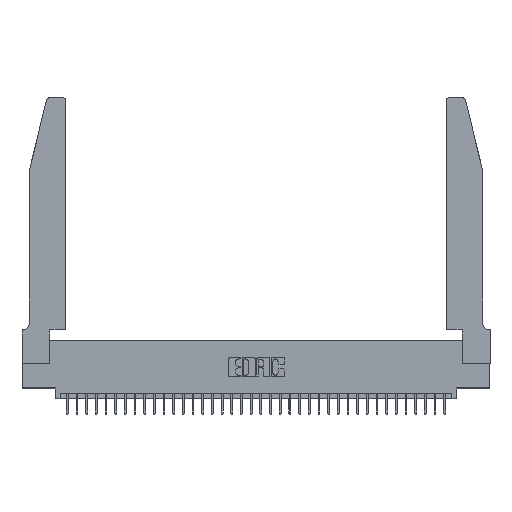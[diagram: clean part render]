
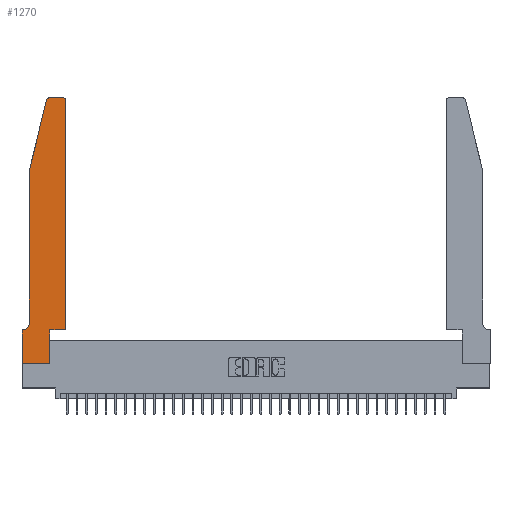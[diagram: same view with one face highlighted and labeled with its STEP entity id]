
A CAD part, top view. The second image highlights one B-rep face of the part: STEP entity #1270.
In plain terms, the highlighted planar face has unit normal (0, 0, 1).
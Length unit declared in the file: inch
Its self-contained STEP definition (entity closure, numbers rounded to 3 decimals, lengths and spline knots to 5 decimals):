
#65 = EDGE_CURVE ( 'NONE', #24321, #22685, #24032, .T. ) ;
#517 = EDGE_CURVE ( 'NONE', #23599, #31405, #6212, .T. ) ;
#1083 = EDGE_CURVE ( 'NONE', #31405, #13949, #21759, .T. ) ;
#1270 = ADVANCED_FACE ( 'NONE', ( #4887 ), #7779, .T. ) ;
#1396 = DIRECTION ( 'NONE',  ( 0., 0., 1. ) ) ;
#2242 = DIRECTION ( 'NONE',  ( 0., -1., 0. ) ) ;
#2376 = VERTEX_POINT ( 'NONE', #35220 ) ;
#2506 = LINE ( 'NONE', #8775, #5583 ) ;
#4100 = ORIENTED_EDGE ( 'NONE', *, *, #517, .T. ) ;
#4130 = EDGE_CURVE ( 'NONE', #23482, #27998, #27490, .T. ) ;
#4410 = EDGE_CURVE ( 'NONE', #2376, #6385, #9303, .T. ) ;
#4876 = LINE ( 'NONE', #26393, #8856 ) ;
#4887 = FACE_OUTER_BOUND ( 'NONE', #32056, .T. ) ;
#5583 = VECTOR ( 'NONE', #20606, 39.37008 ) ;
#5746 = ORIENTED_EDGE ( 'NONE', *, *, #16310, .T. ) ;
#6212 = CIRCLE ( 'NONE', #23201, 0.03 ) ;
#6385 = VERTEX_POINT ( 'NONE', #10218 ) ;
#6633 = VECTOR ( 'NONE', #18311, 39.37008 ) ;
#6755 = ORIENTED_EDGE ( 'NONE', *, *, #4410, .T. ) ;
#6871 = CARTESIAN_POINT ( 'NONE',  ( 0.4205, 2.75, 0.37 ) ) ;
#7328 = LINE ( 'NONE', #31732, #21506 ) ;
#7779 = PLANE ( 'NONE',  #19932 ) ;
#7938 = VECTOR ( 'NONE', #24147, 39.37008 ) ;
#8775 = CARTESIAN_POINT ( 'NONE',  ( 0., 0., 0.37 ) ) ;
#8856 = VECTOR ( 'NONE', #24224, 39.37008 ) ;
#9303 = LINE ( 'NONE', #9521, #28753 ) ;
#9521 = CARTESIAN_POINT ( 'NONE',  ( 0.2865, 0.35, 0.37 ) ) ;
#9936 = CARTESIAN_POINT ( 'NONE',  ( 0.0755, 2., 0.37 ) ) ;
#10218 = CARTESIAN_POINT ( 'NONE',  ( 0.2865, 0.35, 0.37 ) ) ;
#10631 = CARTESIAN_POINT ( 'NONE',  ( 0., 0.35, 0.37 ) ) ;
#10821 = CARTESIAN_POINT ( 'NONE',  ( 0.0055, 0.42, 0.37 ) ) ;
#11237 = CARTESIAN_POINT ( 'NONE',  ( 0.0755, 2., 0.37 ) ) ;
#11319 = EDGE_CURVE ( 'NONE', #13949, #31906, #30739, .T. ) ;
#13082 = ORIENTED_EDGE ( 'NONE', *, *, #11319, .T. ) ;
#13360 = EDGE_CURVE ( 'NONE', #6385, #20041, #4876, .T. ) ;
#13949 = VERTEX_POINT ( 'NONE', #18133 ) ;
#14176 = CARTESIAN_POINT ( 'NONE',  ( 0.284, 2.75, 0.37 ) ) ;
#14812 = DIRECTION ( 'NONE',  ( -1., 0., 0. ) ) ;
#15260 = CARTESIAN_POINT ( 'NONE',  ( 0.4205, 2.72, 0.37 ) ) ;
#15586 = CARTESIAN_POINT ( 'NONE',  ( 0.0755, 0.35, 0.37 ) ) ;
#16310 = EDGE_CURVE ( 'NONE', #19633, #24321, #23368, .T. ) ;
#16917 = ORIENTED_EDGE ( 'NONE', *, *, #17062, .T. ) ;
#17062 = EDGE_CURVE ( 'NONE', #31906, #19633, #22103, .T. ) ;
#17596 = CARTESIAN_POINT ( 'NONE',  ( 0.0055, 0.35, 0.37 ) ) ;
#18133 = CARTESIAN_POINT ( 'NONE',  ( 0.0755, 2., 0.37 ) ) ;
#18311 = DIRECTION ( 'NONE',  ( -0.239, -0.971, 0. ) ) ;
#18563 = ORIENTED_EDGE ( 'NONE', *, *, #35576, .T. ) ;
#19015 = DIRECTION ( 'NONE',  ( 1., 0., 0. ) ) ;
#19085 = CARTESIAN_POINT ( 'NONE',  ( 0.4505, 0.35, 0.37 ) ) ;
#19585 = ORIENTED_EDGE ( 'NONE', *, *, #28231, .T. ) ;
#19633 = VERTEX_POINT ( 'NONE', #17596 ) ;
#19932 = AXIS2_PLACEMENT_3D ( 'NONE', #10631, #30389, #24846 ) ;
#19980 = AXIS2_PLACEMENT_3D ( 'NONE', #15260, #1396, #20960 ) ;
#20041 = VERTEX_POINT ( 'NONE', #28250 ) ;
#20606 = DIRECTION ( 'NONE',  ( 1., 0., 0. ) ) ;
#20960 = DIRECTION ( 'NONE',  ( 1., 0., 0. ) ) ;
#21506 = VECTOR ( 'NONE', #14812, 39.37008 ) ;
#21719 = DIRECTION ( 'NONE',  ( 0., 0., 1. ) ) ;
#21759 = LINE ( 'NONE', #11237, #6633 ) ;
#21863 = VECTOR ( 'NONE', #26965, 39.37008 ) ;
#22103 = CIRCLE ( 'NONE', #25994, 0.07 ) ;
#22685 = VERTEX_POINT ( 'NONE', #27129 ) ;
#23062 = ORIENTED_EDGE ( 'NONE', *, *, #65, .T. ) ;
#23201 = AXIS2_PLACEMENT_3D ( 'NONE', #35935, #21719, #19015 ) ;
#23368 = LINE ( 'NONE', #15586, #7938 ) ;
#23482 = VERTEX_POINT ( 'NONE', #25047 ) ;
#23599 = VERTEX_POINT ( 'NONE', #14176 ) ;
#23753 = VECTOR ( 'NONE', #33496, 39.37008 ) ;
#23777 = CARTESIAN_POINT ( 'NONE',  ( 0.25487, 2.72718, 0.37 ) ) ;
#24032 = LINE ( 'NONE', #35871, #31125 ) ;
#24147 = DIRECTION ( 'NONE',  ( -1., 0., 0. ) ) ;
#24224 = DIRECTION ( 'NONE',  ( 1., 0., 0. ) ) ;
#24321 = VERTEX_POINT ( 'NONE', #36551 ) ;
#24846 = DIRECTION ( 'NONE',  ( 1., 0., 0. ) ) ;
#25047 = CARTESIAN_POINT ( 'NONE',  ( 0.4505, 2.72, 0.37 ) ) ;
#25326 = ORIENTED_EDGE ( 'NONE', *, *, #33164, .T. ) ;
#25994 = AXIS2_PLACEMENT_3D ( 'NONE', #10821, #30830, #33272 ) ;
#26393 = CARTESIAN_POINT ( 'NONE',  ( 0.4505, 0.35, 0.37 ) ) ;
#26965 = DIRECTION ( 'NONE',  ( 0., -1., 0. ) ) ;
#27129 = CARTESIAN_POINT ( 'NONE',  ( 0., 0., 0.37 ) ) ;
#27490 = CIRCLE ( 'NONE', #19980, 0.03 ) ;
#27998 = VERTEX_POINT ( 'NONE', #6871 ) ;
#28231 = EDGE_CURVE ( 'NONE', #20041, #23482, #34776, .T. ) ;
#28250 = CARTESIAN_POINT ( 'NONE',  ( 0.4505, 0.35, 0.37 ) ) ;
#28753 = VECTOR ( 'NONE', #35430, 39.37008 ) ;
#28917 = CARTESIAN_POINT ( 'NONE',  ( 0.0755, 0.42, 0.37 ) ) ;
#30389 = DIRECTION ( 'NONE',  ( 0., 0., 1. ) ) ;
#30739 = LINE ( 'NONE', #9936, #21863 ) ;
#30830 = DIRECTION ( 'NONE',  ( 0., 0., -1. ) ) ;
#31125 = VECTOR ( 'NONE', #2242, 39.37008 ) ;
#31405 = VERTEX_POINT ( 'NONE', #23777 ) ;
#31732 = CARTESIAN_POINT ( 'NONE',  ( 0.2605, 2.75, 0.37 ) ) ;
#31906 = VERTEX_POINT ( 'NONE', #28917 ) ;
#32056 = EDGE_LOOP ( 'NONE', ( #25326, #4100, #34082, #13082, #16917, #5746, #23062, #18563, #6755, #35699, #19585, #32792 ) ) ;
#32792 = ORIENTED_EDGE ( 'NONE', *, *, #4130, .T. ) ;
#33164 = EDGE_CURVE ( 'NONE', #27998, #23599, #7328, .T. ) ;
#33272 = DIRECTION ( 'NONE',  ( -1., 0., 0. ) ) ;
#33496 = DIRECTION ( 'NONE',  ( 0., 1., 0. ) ) ;
#34082 = ORIENTED_EDGE ( 'NONE', *, *, #1083, .T. ) ;
#34776 = LINE ( 'NONE', #19085, #23753 ) ;
#35220 = CARTESIAN_POINT ( 'NONE',  ( 0.2865, 0., 0.37 ) ) ;
#35430 = DIRECTION ( 'NONE',  ( 0., 1., 0. ) ) ;
#35576 = EDGE_CURVE ( 'NONE', #22685, #2376, #2506, .T. ) ;
#35699 = ORIENTED_EDGE ( 'NONE', *, *, #13360, .T. ) ;
#35871 = CARTESIAN_POINT ( 'NONE',  ( 0., 0., 0.37 ) ) ;
#35935 = CARTESIAN_POINT ( 'NONE',  ( 0.284, 2.72, 0.37 ) ) ;
#36551 = CARTESIAN_POINT ( 'NONE',  ( 0., 0.35, 0.37 ) ) ;
